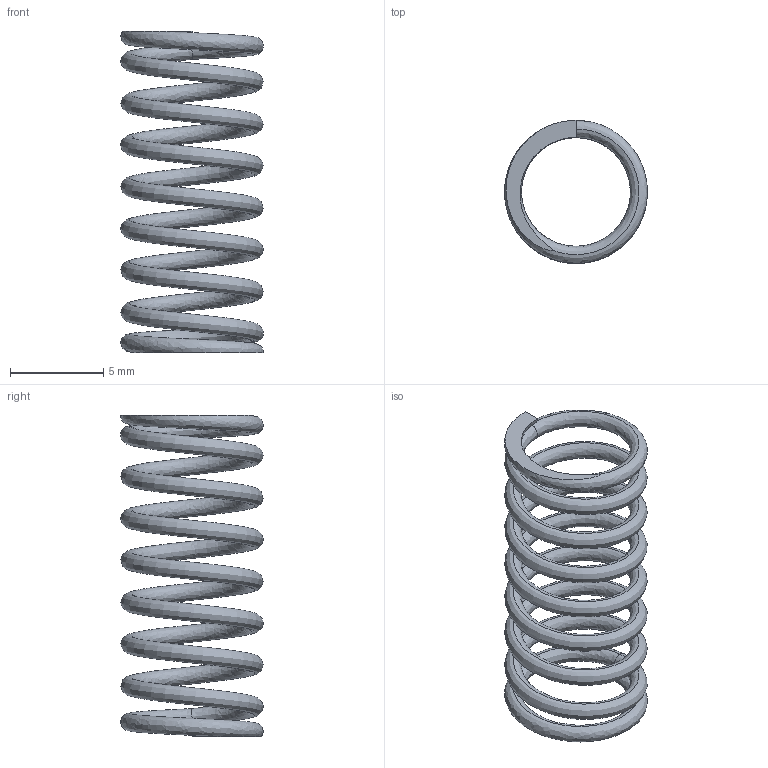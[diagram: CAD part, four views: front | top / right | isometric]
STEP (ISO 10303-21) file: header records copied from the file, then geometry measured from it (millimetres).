
FILE_DESCRIPTION (( 'STEP AP214' ), '1' );
FILE_NAME ('User Library-Telescopic Stock_Telescopic Stock Spring_Installed1.STEP', '2013-05-23T12:57:00', ( 'Asher' ), ( '' ), 'SwSTEP 2.0', 'SolidWorks 2013', '' );
FILE_SCHEMA (( 'AUTOMOTIVE_DESIGN' ));
Length unit declared in the file: millimetre
Products named in the file (1): User Library-Telescopic Stock_Telescopic Stock Spring_Installed1
Bounding box: 7.67 x 7.67 x 17.25 mm (x, y, z)
Volume: 120.3 mm3; surface area: 533.7 mm2
Topology: 1 solids, 1 shells, 10 faces, 20 edges, 12 vertices
Faces by surface type: bspline 6, plane 4
Entity records: 2988 total; most frequent: CARTESIAN_POINT 2813, ORIENTED_EDGE 40, EDGE_CURVE 20, DIRECTION 12, VERTEX_POINT 12, B_SPLINE_CURVE_WITH_KNOTS 10, EDGE_LOOP 10, ADVANCED_FACE 10
